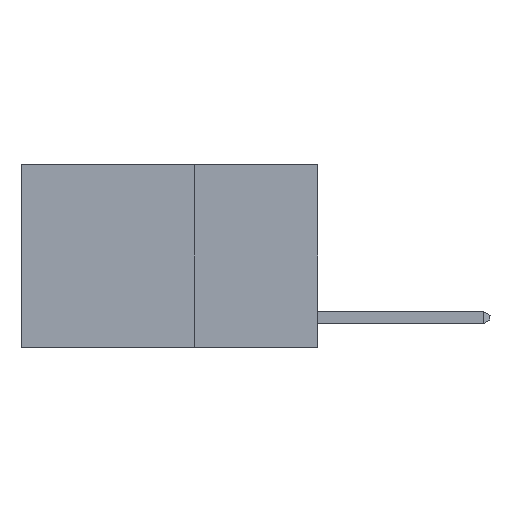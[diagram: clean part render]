
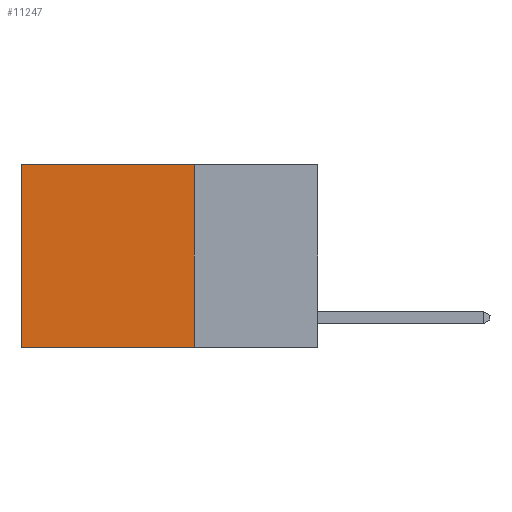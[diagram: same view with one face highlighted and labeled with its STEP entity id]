
A CAD part, left-side view. The second image highlights one B-rep face of the part: STEP entity #11247.
In plain terms, the highlighted planar face has unit normal (-1, 0, 0).
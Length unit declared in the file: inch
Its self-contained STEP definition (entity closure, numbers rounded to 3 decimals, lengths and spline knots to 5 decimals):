
#442 = ORIENTED_EDGE ( 'NONE', *, *, #21174, .T. ) ;
#1440 = VECTOR ( 'NONE', #10527, 39.37008 ) ;
#3146 = VERTEX_POINT ( 'NONE', #7577 ) ;
#3237 = CARTESIAN_POINT ( 'NONE',  ( 0.2625, 0.25, 0. ) ) ;
#3630 = CARTESIAN_POINT ( 'NONE',  ( 0.2625, 0.6, 0. ) ) ;
#4567 = VECTOR ( 'NONE', #13136, 39.37008 ) ;
#4689 = CARTESIAN_POINT ( 'NONE',  ( 0.2625, 0.25, 0. ) ) ;
#4830 = DIRECTION ( 'NONE',  ( 1., 0., 0. ) ) ;
#4977 = CARTESIAN_POINT ( 'NONE',  ( 0.2625, 0.6, 0. ) ) ;
#5267 = DIRECTION ( 'NONE',  ( 0., 0., -1. ) ) ;
#5281 = ORIENTED_EDGE ( 'NONE', *, *, #20416, .F. ) ;
#5518 = AXIS2_PLACEMENT_3D ( 'NONE', #4689, #4830, #6522 ) ;
#6338 = VERTEX_POINT ( 'NONE', #19466 ) ;
#6522 = DIRECTION ( 'NONE',  ( 0., 0., -1. ) ) ;
#6858 = FACE_OUTER_BOUND ( 'NONE', #11365, .T. ) ;
#7577 = CARTESIAN_POINT ( 'NONE',  ( 0.2625, 0.25, 0. ) ) ;
#8389 = PLANE ( 'NONE',  #5518 ) ;
#9316 = VECTOR ( 'NONE', #14285, 39.37008 ) ;
#10095 = LINE ( 'NONE', #19496, #9316 ) ;
#10527 = DIRECTION ( 'NONE',  ( 0., 0., -1. ) ) ;
#11203 = LINE ( 'NONE', #4977, #15235 ) ;
#11247 = ADVANCED_FACE ( 'NONE', ( #6858 ), #8389, .F. ) ;
#11365 = EDGE_LOOP ( 'NONE', ( #442, #13266, #5281, #17049 ) ) ;
#12082 = EDGE_CURVE ( 'NONE', #6338, #14384, #10095, .T. ) ;
#12348 = CARTESIAN_POINT ( 'NONE',  ( 0.2625, 0.25, 0. ) ) ;
#13136 = DIRECTION ( 'NONE',  ( 0., 1., 0. ) ) ;
#13266 = ORIENTED_EDGE ( 'NONE', *, *, #12082, .F. ) ;
#14285 = DIRECTION ( 'NONE',  ( 0., 1., 0. ) ) ;
#14384 = VERTEX_POINT ( 'NONE', #21011 ) ;
#15235 = VECTOR ( 'NONE', #5267, 39.37008 ) ;
#16748 = LINE ( 'NONE', #3237, #4567 ) ;
#17049 = ORIENTED_EDGE ( 'NONE', *, *, #21807, .T. ) ;
#17895 = LINE ( 'NONE', #12348, #1440 ) ;
#18034 = VERTEX_POINT ( 'NONE', #3630 ) ;
#19466 = CARTESIAN_POINT ( 'NONE',  ( 0.2625, 0.25, -0.37 ) ) ;
#19496 = CARTESIAN_POINT ( 'NONE',  ( 0.2625, 0.25, -0.37 ) ) ;
#20416 = EDGE_CURVE ( 'NONE', #3146, #6338, #17895, .T. ) ;
#21011 = CARTESIAN_POINT ( 'NONE',  ( 0.2625, 0.6, -0.37 ) ) ;
#21174 = EDGE_CURVE ( 'NONE', #18034, #14384, #11203, .T. ) ;
#21807 = EDGE_CURVE ( 'NONE', #3146, #18034, #16748, .T. ) ;
